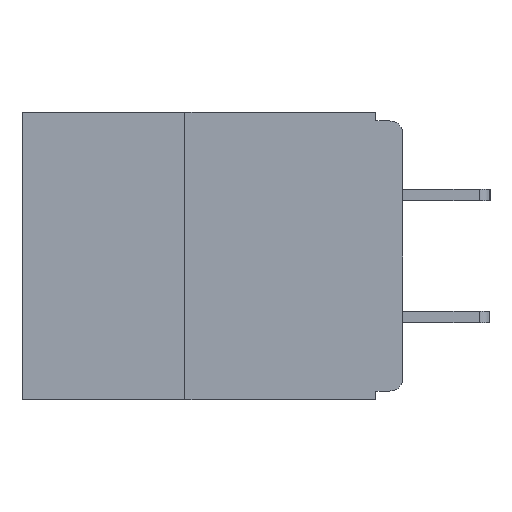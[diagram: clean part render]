
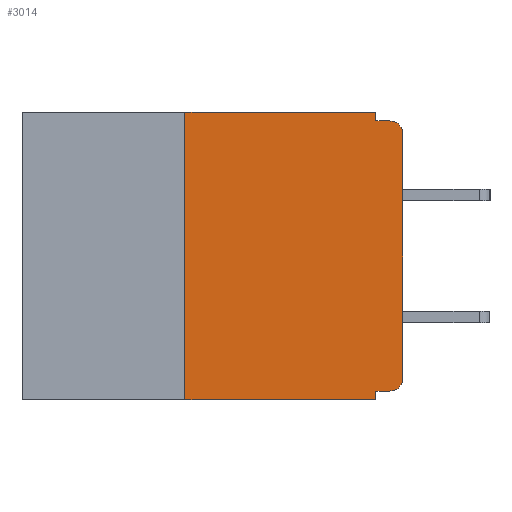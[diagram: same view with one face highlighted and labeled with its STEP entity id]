
A CAD part, left-side view. The second image highlights one B-rep face of the part: STEP entity #3014.
In plain terms, the highlighted planar face has unit normal (-1, 0, 0).
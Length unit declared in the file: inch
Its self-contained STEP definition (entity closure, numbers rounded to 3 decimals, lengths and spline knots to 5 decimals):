
#434 = LINE ( 'NONE', #10764, #11084 ) ;
#780 = CARTESIAN_POINT ( 'NONE',  ( 0., 0.437, 0. ) ) ;
#1151 = VECTOR ( 'NONE', #2230, 39.37008 ) ;
#1179 = EDGE_CURVE ( 'NONE', #10606, #6235, #5555, .T. ) ;
#1217 = EDGE_CURVE ( 'NONE', #6235, #12806, #8360, .T. ) ;
#1218 = ORIENTED_EDGE ( 'NONE', *, *, #1217, .T. ) ;
#1854 = EDGE_CURVE ( 'NONE', #11553, #10606, #6368, .T. ) ;
#1912 = VERTEX_POINT ( 'NONE', #3976 ) ;
#1930 = ORIENTED_EDGE ( 'NONE', *, *, #6440, .F. ) ;
#2073 = DIRECTION ( 'NONE',  ( -1., 0., 0. ) ) ;
#2191 = VERTEX_POINT ( 'NONE', #9442 ) ;
#2192 = FACE_OUTER_BOUND ( 'NONE', #4602, .T. ) ;
#2230 = DIRECTION ( 'NONE',  ( 0., -1., 0. ) ) ;
#2330 = VERTEX_POINT ( 'NONE', #4969 ) ;
#2395 = CARTESIAN_POINT ( 'NONE',  ( 0., 0.015, -0.305 ) ) ;
#2628 = CARTESIAN_POINT ( 'NONE',  ( 0., 0.031, -0.33 ) ) ;
#2639 = DIRECTION ( 'NONE',  ( 0., 0., 1. ) ) ;
#2688 = CARTESIAN_POINT ( 'NONE',  ( 0., 0.437, -0.33 ) ) ;
#2997 = CARTESIAN_POINT ( 'NONE',  ( 0., 0.015, -0.025 ) ) ;
#3014 = ADVANCED_FACE ( 'NONE', ( #2192 ), #4201, .F. ) ;
#3180 = CARTESIAN_POINT ( 'NONE',  ( 0., 0., -0.025 ) ) ;
#3300 = CARTESIAN_POINT ( 'NONE',  ( 0., 0.031, -0.33 ) ) ;
#3384 = DIRECTION ( 'NONE',  ( 0., 0., -1. ) ) ;
#3496 = VERTEX_POINT ( 'NONE', #9109 ) ;
#3531 = DIRECTION ( 'NONE',  ( -1., 0., 0. ) ) ;
#3587 = DIRECTION ( 'NONE',  ( 0., 0., 1. ) ) ;
#3692 = CARTESIAN_POINT ( 'NONE',  ( 0., 0., -0.01 ) ) ;
#3729 = CARTESIAN_POINT ( 'NONE',  ( 0., 0.25, 0. ) ) ;
#3976 = CARTESIAN_POINT ( 'NONE',  ( 0., 0.031, -0.01 ) ) ;
#4005 = EDGE_CURVE ( 'NONE', #1912, #12806, #12612, .T. ) ;
#4201 = PLANE ( 'NONE',  #11616 ) ;
#4463 = VERTEX_POINT ( 'NONE', #3300 ) ;
#4599 = EDGE_CURVE ( 'NONE', #3496, #4463, #8168, .T. ) ;
#4602 = EDGE_LOOP ( 'NONE', ( #8393, #1218, #4798, #11011, #11628, #12838, #12682, #8553, #1930, #11033 ) ) ;
#4620 = AXIS2_PLACEMENT_3D ( 'NONE', #2997, #3531, #3384 ) ;
#4798 = ORIENTED_EDGE ( 'NONE', *, *, #4005, .F. ) ;
#4969 = CARTESIAN_POINT ( 'NONE',  ( 0., 0.031, 0. ) ) ;
#5231 = EDGE_CURVE ( 'NONE', #8128, #2330, #434, .T. ) ;
#5542 = DIRECTION ( 'NONE',  ( 0., -1., 0. ) ) ;
#5555 = LINE ( 'NONE', #7041, #5897 ) ;
#5765 = CARTESIAN_POINT ( 'NONE',  ( 0., 0., -0.305 ) ) ;
#5897 = VECTOR ( 'NONE', #2639, 39.37008 ) ;
#6235 = VERTEX_POINT ( 'NONE', #3180 ) ;
#6368 = CIRCLE ( 'NONE', #13240, 0.015 ) ;
#6440 = EDGE_CURVE ( 'NONE', #11553, #3496, #12566, .T. ) ;
#6452 = CARTESIAN_POINT ( 'NONE',  ( 0., 0.015, -0.01 ) ) ;
#6842 = EDGE_CURVE ( 'NONE', #2330, #1912, #10246, .T. ) ;
#6964 = VECTOR ( 'NONE', #3587, 39.37008 ) ;
#7041 = CARTESIAN_POINT ( 'NONE',  ( 0., 0., 0. ) ) ;
#7099 = VECTOR ( 'NONE', #10424, 39.37008 ) ;
#8128 = VERTEX_POINT ( 'NONE', #3729 ) ;
#8168 = LINE ( 'NONE', #2628, #10635 ) ;
#8189 = EDGE_CURVE ( 'NONE', #2191, #4463, #10207, .T. ) ;
#8360 = CIRCLE ( 'NONE', #4620, 0.015 ) ;
#8393 = ORIENTED_EDGE ( 'NONE', *, *, #1179, .T. ) ;
#8553 = ORIENTED_EDGE ( 'NONE', *, *, #4599, .F. ) ;
#9109 = CARTESIAN_POINT ( 'NONE',  ( 0., 0.031, -0.32 ) ) ;
#9218 = DIRECTION ( 'NONE',  ( 0., 0., -1. ) ) ;
#9442 = CARTESIAN_POINT ( 'NONE',  ( 0., 0.25, -0.33 ) ) ;
#9909 = CARTESIAN_POINT ( 'NONE',  ( 0., 0.25, -0.33 ) ) ;
#10113 = DIRECTION ( 'NONE',  ( 0., -1., 0. ) ) ;
#10178 = DIRECTION ( 'NONE',  ( 0., 0., -1. ) ) ;
#10207 = LINE ( 'NONE', #2688, #12522 ) ;
#10246 = LINE ( 'NONE', #12466, #12867 ) ;
#10424 = DIRECTION ( 'NONE',  ( 0., 1., 0. ) ) ;
#10549 = DIRECTION ( 'NONE',  ( 1., 0., 0. ) ) ;
#10598 = CARTESIAN_POINT ( 'NONE',  ( 0., 0.015, -0.32 ) ) ;
#10606 = VERTEX_POINT ( 'NONE', #5765 ) ;
#10635 = VECTOR ( 'NONE', #11150, 39.37008 ) ;
#10666 = CARTESIAN_POINT ( 'NONE',  ( 0., 0., -0.32 ) ) ;
#10764 = CARTESIAN_POINT ( 'NONE',  ( 0., 0.437, 0. ) ) ;
#11011 = ORIENTED_EDGE ( 'NONE', *, *, #6842, .F. ) ;
#11033 = ORIENTED_EDGE ( 'NONE', *, *, #1854, .T. ) ;
#11084 = VECTOR ( 'NONE', #5542, 39.37008 ) ;
#11150 = DIRECTION ( 'NONE',  ( 0., 0., -1. ) ) ;
#11553 = VERTEX_POINT ( 'NONE', #10598 ) ;
#11616 = AXIS2_PLACEMENT_3D ( 'NONE', #780, #10549, #9218 ) ;
#11628 = ORIENTED_EDGE ( 'NONE', *, *, #5231, .F. ) ;
#11856 = LINE ( 'NONE', #9909, #6964 ) ;
#12379 = EDGE_CURVE ( 'NONE', #2191, #8128, #11856, .T. ) ;
#12466 = CARTESIAN_POINT ( 'NONE',  ( 0., 0.031, 0. ) ) ;
#12522 = VECTOR ( 'NONE', #10113, 39.37008 ) ;
#12566 = LINE ( 'NONE', #10666, #7099 ) ;
#12612 = LINE ( 'NONE', #3692, #1151 ) ;
#12682 = ORIENTED_EDGE ( 'NONE', *, *, #8189, .T. ) ;
#12742 = DIRECTION ( 'NONE',  ( 0., 0., -1. ) ) ;
#12806 = VERTEX_POINT ( 'NONE', #6452 ) ;
#12838 = ORIENTED_EDGE ( 'NONE', *, *, #12379, .F. ) ;
#12867 = VECTOR ( 'NONE', #12742, 39.37008 ) ;
#13240 = AXIS2_PLACEMENT_3D ( 'NONE', #2395, #2073, #10178 ) ;
